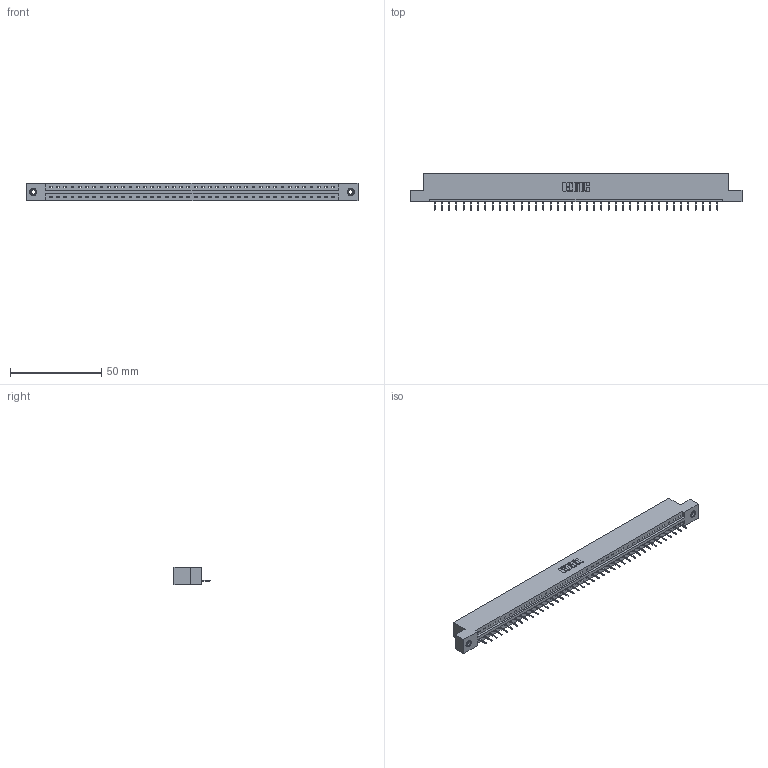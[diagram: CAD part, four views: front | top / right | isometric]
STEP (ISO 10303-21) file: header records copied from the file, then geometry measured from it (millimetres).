
FILE_DESCRIPTION (( 'STEP AP203' ), '1' );
FILE_NAME ('387-040-524-107.STEP', '2019-10-04T18:37:20', ( '' ), ( '' ), 'SwSTEP 2.0', 'SolidWorks 2016', '' );
FILE_SCHEMA (( 'CONFIG_CONTROL_DESIGN' ));
Length unit declared in the file: inch
Products named in the file (4): 345-250-001_345-250-005-103; 345-292-001_345-293-124; 337 Part_Flush Mounting Lugs - 0.156 Dia-TI; 387-040-524-107
Assembly tree (43 placements, depth 2):
  387-040-524-107
    337 Part_Flush Mounting Lugs - 0.156 Dia-TI
    345-292-001_345-293-124  x40
    345-250-001_345-250-005-103  x2
Bounding box: 181.51 x 19.69 x 9.4 mm (x, y, z)
Volume: 18668.2 mm3; surface area: 18765.1 mm2
Topology: 43 solids, 43 shells, 2814 faces, 8127 edges, 5250 vertices
Faces by surface type: plane 2182, cylinder 616, cone 12, torus 4
Entity records: 31252 total; most frequent: CARTESIAN_POINT 5421, ORIENTED_EDGE 5390, DIRECTION 4601, EDGE_CURVE 2695, LINE 2551, VECTOR 2551, VERTEX_POINT 1788, AXIS2_PLACEMENT_3D 1025
